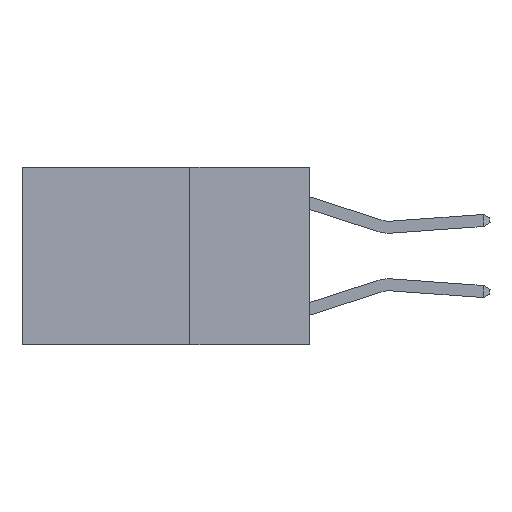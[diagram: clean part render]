
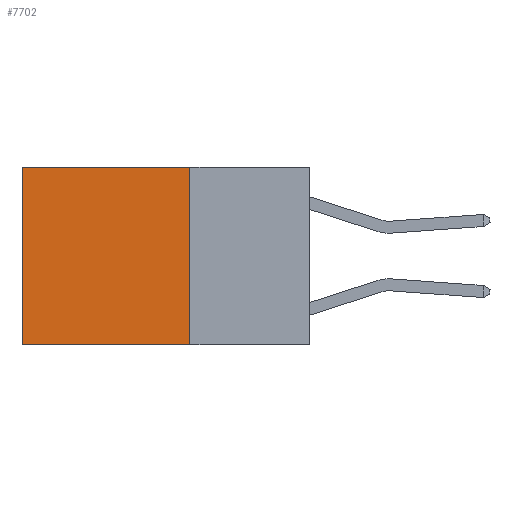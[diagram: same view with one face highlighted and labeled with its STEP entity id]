
A CAD part, left-side view. The second image highlights one B-rep face of the part: STEP entity #7702.
In plain terms, the highlighted planar face has unit normal (-1, 0, 0).
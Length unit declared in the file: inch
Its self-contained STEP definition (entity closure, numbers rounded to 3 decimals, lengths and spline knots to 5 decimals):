
#572 = VECTOR ( 'NONE', #10800, 39.37008 ) ;
#817 = VECTOR ( 'NONE', #10746, 39.37008 ) ;
#909 = LINE ( 'NONE', #1680, #2245 ) ;
#1680 = CARTESIAN_POINT ( 'NONE',  ( 0.2625, 0.25, -0.37 ) ) ;
#1795 = CARTESIAN_POINT ( 'NONE',  ( 0.2625, 0.6, -0.37 ) ) ;
#1843 = FACE_OUTER_BOUND ( 'NONE', #6874, .T. ) ;
#1868 = VERTEX_POINT ( 'NONE', #5419 ) ;
#1892 = LINE ( 'NONE', #5750, #817 ) ;
#1909 = PLANE ( 'NONE',  #7473 ) ;
#2219 = CARTESIAN_POINT ( 'NONE',  ( 0.2625, 0.25, 0. ) ) ;
#2245 = VECTOR ( 'NONE', #4583, 39.37008 ) ;
#2957 = ORIENTED_EDGE ( 'NONE', *, *, #5231, .T. ) ;
#3802 = DIRECTION ( 'NONE',  ( 0., 0., -1. ) ) ;
#3886 = LINE ( 'NONE', #4642, #8121 ) ;
#3911 = CARTESIAN_POINT ( 'NONE',  ( 0.2625, 0.25, 0. ) ) ;
#4220 = EDGE_CURVE ( 'NONE', #1868, #5970, #909, .T. ) ;
#4583 = DIRECTION ( 'NONE',  ( 0., 1., 0. ) ) ;
#4642 = CARTESIAN_POINT ( 'NONE',  ( 0.2625, 0.25, 0. ) ) ;
#5231 = EDGE_CURVE ( 'NONE', #12429, #10421, #8949, .T. ) ;
#5419 = CARTESIAN_POINT ( 'NONE',  ( 0.2625, 0.25, -0.37 ) ) ;
#5750 = CARTESIAN_POINT ( 'NONE',  ( 0.2625, 0.6, 0. ) ) ;
#5970 = VERTEX_POINT ( 'NONE', #1795 ) ;
#6874 = EDGE_LOOP ( 'NONE', ( #9460, #10562, #11518, #2957 ) ) ;
#7473 = AXIS2_PLACEMENT_3D ( 'NONE', #10385, #12212, #3802 ) ;
#7545 = DIRECTION ( 'NONE',  ( 0., 0., -1. ) ) ;
#7702 = ADVANCED_FACE ( 'NONE', ( #1843 ), #1909, .F. ) ;
#8121 = VECTOR ( 'NONE', #7545, 39.37008 ) ;
#8403 = EDGE_CURVE ( 'NONE', #10421, #5970, #1892, .T. ) ;
#8949 = LINE ( 'NONE', #3911, #572 ) ;
#9460 = ORIENTED_EDGE ( 'NONE', *, *, #8403, .T. ) ;
#10385 = CARTESIAN_POINT ( 'NONE',  ( 0.2625, 0.25, 0. ) ) ;
#10421 = VERTEX_POINT ( 'NONE', #12030 ) ;
#10562 = ORIENTED_EDGE ( 'NONE', *, *, #4220, .F. ) ;
#10566 = EDGE_CURVE ( 'NONE', #12429, #1868, #3886, .T. ) ;
#10746 = DIRECTION ( 'NONE',  ( 0., 0., -1. ) ) ;
#10800 = DIRECTION ( 'NONE',  ( 0., 1., 0. ) ) ;
#11518 = ORIENTED_EDGE ( 'NONE', *, *, #10566, .F. ) ;
#12030 = CARTESIAN_POINT ( 'NONE',  ( 0.2625, 0.6, 0. ) ) ;
#12212 = DIRECTION ( 'NONE',  ( 1., 0., 0. ) ) ;
#12429 = VERTEX_POINT ( 'NONE', #2219 ) ;
